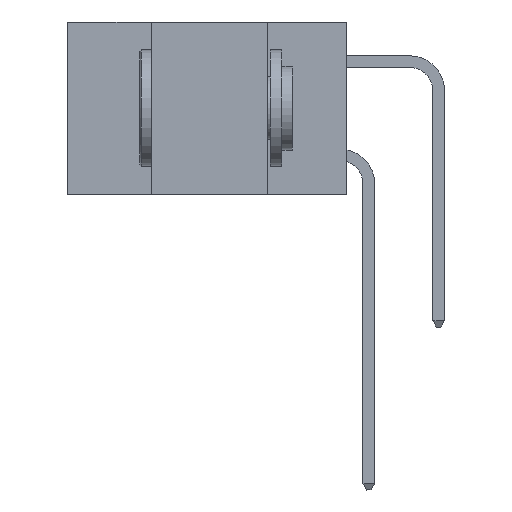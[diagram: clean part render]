
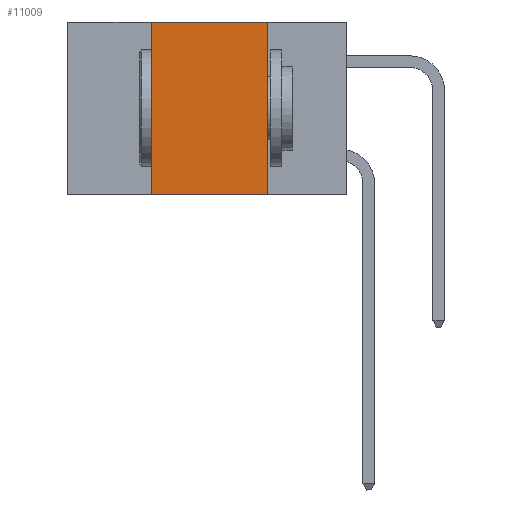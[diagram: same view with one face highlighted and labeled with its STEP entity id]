
A CAD part, left-side view. The second image highlights one B-rep face of the part: STEP entity #11009.
In plain terms, the highlighted planar face has unit normal (-1, 0, 0).
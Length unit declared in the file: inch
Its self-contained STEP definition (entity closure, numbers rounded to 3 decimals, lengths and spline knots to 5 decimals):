
#670 = ORIENTED_EDGE ( 'NONE', *, *, #6229, .T. ) ;
#1576 = EDGE_CURVE ( 'NONE', #3103, #13593, #18278, .T. ) ;
#1851 = ORIENTED_EDGE ( 'NONE', *, *, #1576, .F. ) ;
#2012 = VECTOR ( 'NONE', #8533, 39.37008 ) ;
#2150 = EDGE_LOOP ( 'NONE', ( #18297, #19362, #1851, #670 ) ) ;
#3001 = VERTEX_POINT ( 'NONE', #7459 ) ;
#3103 = VERTEX_POINT ( 'NONE', #10302 ) ;
#3959 = DIRECTION ( 'NONE',  ( 0., -1., 0. ) ) ;
#4916 = VECTOR ( 'NONE', #16963, 39.37008 ) ;
#5551 = VERTEX_POINT ( 'NONE', #13643 ) ;
#5690 = CARTESIAN_POINT ( 'NONE',  ( 0., 0.6, 0. ) ) ;
#6229 = EDGE_CURVE ( 'NONE', #3103, #5551, #15029, .T. ) ;
#6677 = CARTESIAN_POINT ( 'NONE',  ( 0., 0.42, 0. ) ) ;
#7336 = CARTESIAN_POINT ( 'NONE',  ( 0., 0.17, 0. ) ) ;
#7459 = CARTESIAN_POINT ( 'NONE',  ( 0., 0.17, 0. ) ) ;
#8533 = DIRECTION ( 'NONE',  ( 0., 0., 1. ) ) ;
#8752 = PLANE ( 'NONE',  #10112 ) ;
#8910 = DIRECTION ( 'NONE',  ( 0., -1., 0. ) ) ;
#10112 = AXIS2_PLACEMENT_3D ( 'NONE', #13549, #20224, #10393 ) ;
#10228 = CARTESIAN_POINT ( 'NONE',  ( 0., 0.6, -0.37 ) ) ;
#10302 = CARTESIAN_POINT ( 'NONE',  ( 0., 0.42, -0.37 ) ) ;
#10393 = DIRECTION ( 'NONE',  ( 0., 0., -1. ) ) ;
#10945 = VECTOR ( 'NONE', #3959, 39.37008 ) ;
#11009 = ADVANCED_FACE ( 'NONE', ( #17227 ), #8752, .F. ) ;
#13105 = EDGE_CURVE ( 'NONE', #3001, #5551, #14071, .T. ) ;
#13549 = CARTESIAN_POINT ( 'NONE',  ( 0., 0.6, 0. ) ) ;
#13593 = VERTEX_POINT ( 'NONE', #6677 ) ;
#13643 = CARTESIAN_POINT ( 'NONE',  ( 0., 0.17, -0.37 ) ) ;
#14071 = LINE ( 'NONE', #7336, #4916 ) ;
#14678 = VECTOR ( 'NONE', #8910, 39.37008 ) ;
#15029 = LINE ( 'NONE', #10228, #10945 ) ;
#16963 = DIRECTION ( 'NONE',  ( 0., 0., -1. ) ) ;
#17227 = FACE_OUTER_BOUND ( 'NONE', #2150, .T. ) ;
#18278 = LINE ( 'NONE', #18357, #2012 ) ;
#18297 = ORIENTED_EDGE ( 'NONE', *, *, #13105, .F. ) ;
#18357 = CARTESIAN_POINT ( 'NONE',  ( 0., 0.42, 0. ) ) ;
#19183 = EDGE_CURVE ( 'NONE', #13593, #3001, #19536, .T. ) ;
#19362 = ORIENTED_EDGE ( 'NONE', *, *, #19183, .F. ) ;
#19536 = LINE ( 'NONE', #5690, #14678 ) ;
#20224 = DIRECTION ( 'NONE',  ( 1., 0., 0. ) ) ;
